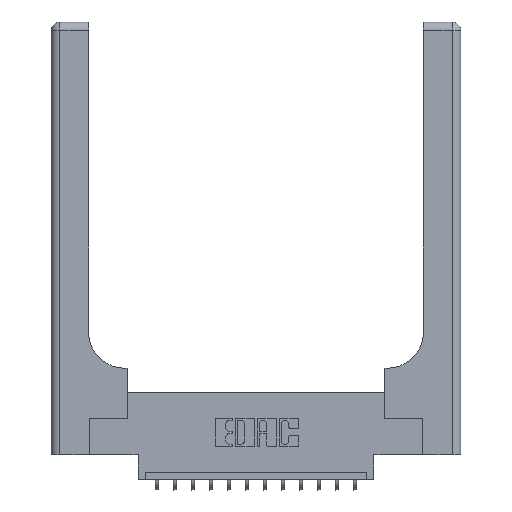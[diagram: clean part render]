
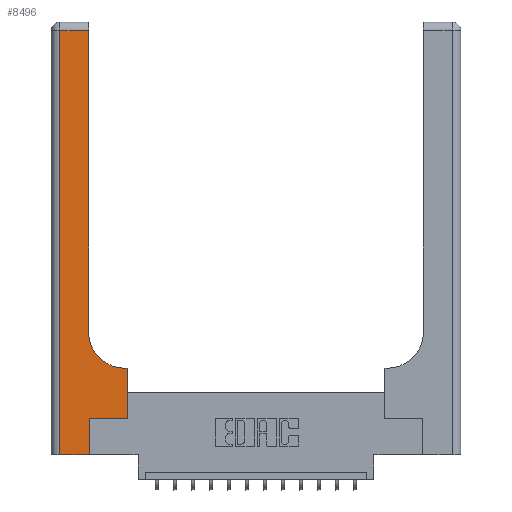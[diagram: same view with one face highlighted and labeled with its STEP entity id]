
A CAD part, top view. The second image highlights one B-rep face of the part: STEP entity #8496.
In plain terms, the highlighted planar face has unit normal (0, 0, 1).
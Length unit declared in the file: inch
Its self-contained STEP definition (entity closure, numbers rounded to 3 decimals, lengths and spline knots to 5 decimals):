
#227 = DIRECTION ( 'NONE',  ( 1., 0., 0. ) ) ;
#303 = CIRCLE ( 'NONE', #9825, 0.25 ) ;
#603 = CARTESIAN_POINT ( 'NONE',  ( 0.26, 0.6, 0.37 ) ) ;
#642 = ORIENTED_EDGE ( 'NONE', *, *, #8561, .T. ) ;
#659 = ORIENTED_EDGE ( 'NONE', *, *, #10156, .T. ) ;
#880 = VECTOR ( 'NONE', #14315, 39.37008 ) ;
#972 = ORIENTED_EDGE ( 'NONE', *, *, #9094, .T. ) ;
#1199 = CARTESIAN_POINT ( 'NONE',  ( 0., 3., 0.37 ) ) ;
#1286 = FACE_OUTER_BOUND ( 'NONE', #4972, .T. ) ;
#1566 = LINE ( 'NONE', #13485, #17073 ) ;
#1631 = DIRECTION ( 'NONE',  ( 1., 0., 0. ) ) ;
#2521 = DIRECTION ( 'NONE',  ( -1., 0., 0. ) ) ;
#3883 = CARTESIAN_POINT ( 'NONE',  ( 0.51, 0.6, 0.37 ) ) ;
#4007 = VERTEX_POINT ( 'NONE', #10523 ) ;
#4016 = PLANE ( 'NONE',  #16016 ) ;
#4078 = EDGE_CURVE ( 'NONE', #9670, #4891, #1566, .T. ) ;
#4189 = LINE ( 'NONE', #9517, #13937 ) ;
#4230 = DIRECTION ( 'NONE',  ( 0., 1., 0. ) ) ;
#4281 = VERTEX_POINT ( 'NONE', #5089 ) ;
#4315 = CARTESIAN_POINT ( 'NONE',  ( 0.26, 3., 0.37 ) ) ;
#4321 = VECTOR ( 'NONE', #4230, 39.37008 ) ;
#4737 = CARTESIAN_POINT ( 'NONE',  ( 0.51, 0.85, 0.37 ) ) ;
#4891 = VERTEX_POINT ( 'NONE', #14022 ) ;
#4972 = EDGE_LOOP ( 'NONE', ( #13595, #14584, #13193, #972, #642, #8513, #9666, #659, #14059 ) ) ;
#5047 = DIRECTION ( 'NONE',  ( -1., 0., 0. ) ) ;
#5089 = CARTESIAN_POINT ( 'NONE',  ( 0.26, 0.85, 0.37 ) ) ;
#5909 = EDGE_CURVE ( 'NONE', #6255, #9670, #11522, .T. ) ;
#5918 = CARTESIAN_POINT ( 'NONE',  ( 0.06, 2.94, 0.37 ) ) ;
#6255 = VERTEX_POINT ( 'NONE', #13770 ) ;
#6635 = DIRECTION ( 'NONE',  ( 0., 1., 0. ) ) ;
#6791 = EDGE_CURVE ( 'NONE', #12793, #4281, #303, .T. ) ;
#6834 = VECTOR ( 'NONE', #11565, 39.37008 ) ;
#7196 = EDGE_CURVE ( 'NONE', #8297, #17206, #15716, .T. ) ;
#7644 = VECTOR ( 'NONE', #6635, 39.37008 ) ;
#8034 = CARTESIAN_POINT ( 'NONE',  ( 0.265, 0., 0.37 ) ) ;
#8297 = VERTEX_POINT ( 'NONE', #9697 ) ;
#8388 = CARTESIAN_POINT ( 'NONE',  ( 0.528, 0.6, 0.37 ) ) ;
#8496 = ADVANCED_FACE ( 'NONE', ( #1286 ), #4016, .F. ) ;
#8513 = ORIENTED_EDGE ( 'NONE', *, *, #16024, .T. ) ;
#8561 = EDGE_CURVE ( 'NONE', #4007, #14213, #9258, .T. ) ;
#9094 = EDGE_CURVE ( 'NONE', #4891, #4007, #16435, .T. ) ;
#9258 = LINE ( 'NONE', #8034, #7644 ) ;
#9517 = CARTESIAN_POINT ( 'NONE',  ( 0.265, 0.25, 0.37 ) ) ;
#9666 = ORIENTED_EDGE ( 'NONE', *, *, #7196, .T. ) ;
#9670 = VERTEX_POINT ( 'NONE', #5918 ) ;
#9697 = CARTESIAN_POINT ( 'NONE',  ( 0.528, 0.25, 0.37 ) ) ;
#9825 = AXIS2_PLACEMENT_3D ( 'NONE', #4737, #12684, #15669 ) ;
#10156 = EDGE_CURVE ( 'NONE', #17206, #12793, #15413, .T. ) ;
#10523 = CARTESIAN_POINT ( 'NONE',  ( 0.265, 0., 0.37 ) ) ;
#10569 = DIRECTION ( 'NONE',  ( 0., 0., -1. ) ) ;
#10654 = VECTOR ( 'NONE', #5047, 39.37008 ) ;
#11522 = LINE ( 'NONE', #16762, #10654 ) ;
#11565 = DIRECTION ( 'NONE',  ( -1., 0., 0. ) ) ;
#11685 = EDGE_CURVE ( 'NONE', #4281, #6255, #16208, .T. ) ;
#12254 = DIRECTION ( 'NONE',  ( 0., -1., 0. ) ) ;
#12684 = DIRECTION ( 'NONE',  ( 0., 0., -1. ) ) ;
#12793 = VERTEX_POINT ( 'NONE', #3883 ) ;
#12818 = CARTESIAN_POINT ( 'NONE',  ( 0.528, 0.25, 0.37 ) ) ;
#13193 = ORIENTED_EDGE ( 'NONE', *, *, #4078, .T. ) ;
#13485 = CARTESIAN_POINT ( 'NONE',  ( 0.06, 3., 0.37 ) ) ;
#13595 = ORIENTED_EDGE ( 'NONE', *, *, #11685, .T. ) ;
#13635 = CARTESIAN_POINT ( 'NONE',  ( 0., 0., 0.37 ) ) ;
#13770 = CARTESIAN_POINT ( 'NONE',  ( 0.26, 2.94, 0.37 ) ) ;
#13937 = VECTOR ( 'NONE', #227, 39.37008 ) ;
#14011 = CARTESIAN_POINT ( 'NONE',  ( 0.265, 0.25, 0.37 ) ) ;
#14022 = CARTESIAN_POINT ( 'NONE',  ( 0.06, 0., 0.37 ) ) ;
#14059 = ORIENTED_EDGE ( 'NONE', *, *, #6791, .T. ) ;
#14213 = VERTEX_POINT ( 'NONE', #14011 ) ;
#14315 = DIRECTION ( 'NONE',  ( 0., 1., 0. ) ) ;
#14346 = VECTOR ( 'NONE', #1631, 39.37008 ) ;
#14584 = ORIENTED_EDGE ( 'NONE', *, *, #5909, .T. ) ;
#15413 = LINE ( 'NONE', #603, #6834 ) ;
#15669 = DIRECTION ( 'NONE',  ( 1., 0., 0. ) ) ;
#15716 = LINE ( 'NONE', #12818, #880 ) ;
#16016 = AXIS2_PLACEMENT_3D ( 'NONE', #1199, #10569, #2521 ) ;
#16024 = EDGE_CURVE ( 'NONE', #14213, #8297, #4189, .T. ) ;
#16208 = LINE ( 'NONE', #4315, #4321 ) ;
#16435 = LINE ( 'NONE', #13635, #14346 ) ;
#16762 = CARTESIAN_POINT ( 'NONE',  ( 0., 2.94, 0.37 ) ) ;
#17073 = VECTOR ( 'NONE', #12254, 39.37008 ) ;
#17206 = VERTEX_POINT ( 'NONE', #8388 ) ;
